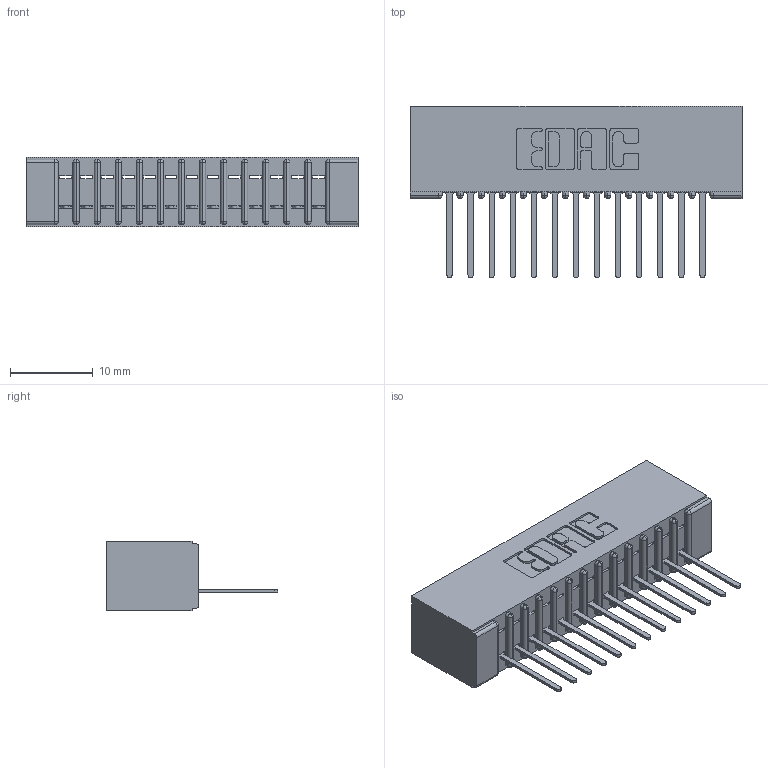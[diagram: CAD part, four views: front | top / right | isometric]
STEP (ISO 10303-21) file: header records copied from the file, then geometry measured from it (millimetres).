
FILE_DESCRIPTION (( 'STEP AP203' ), '1' );
FILE_NAME ('391-013-522-101.STEP', '2018-08-08T16:49:55', ( '' ), ( '' ), 'SwSTEP 2.0', 'SolidWorks 2016', '' );
FILE_SCHEMA (( 'CONFIG_CONTROL_DESIGN' ));
Length unit declared in the file: inch
Products named in the file (3): 341 Part_No Mounting Lugs; 341-292-001_341-292-122; 391-013-522-101
Assembly tree (14 placements, depth 2):
  391-013-522-101
    341 Part_No Mounting Lugs
    341-292-001_341-292-122  x13
Bounding box: 40.01 x 20.62 x 8.38 mm (x, y, z)
Volume: 2355.7 mm3; surface area: 4520.6 mm2
Topology: 14 solids, 14 shells, 1174 faces, 3373 edges, 2166 vertices
Faces by surface type: plane 727, cylinder 395, sphere 28, torus 24
Entity records: 18902 total; most frequent: CARTESIAN_POINT 3198, ORIENTED_EDGE 3186, DIRECTION 3109, EDGE_CURVE 1593, VECTOR 1259, LINE 1259, VERTEX_POINT 1014, AXIS2_PLACEMENT_3D 925
